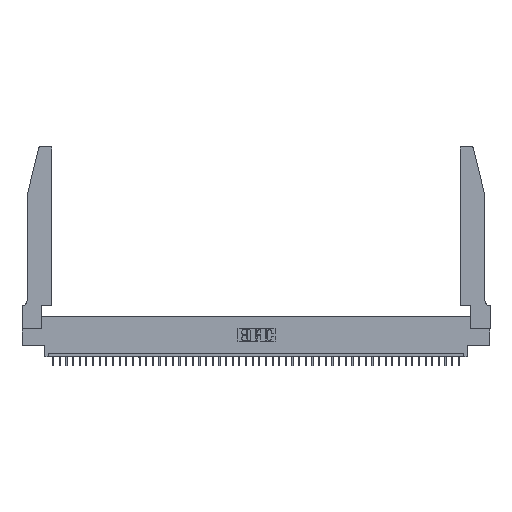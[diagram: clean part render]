
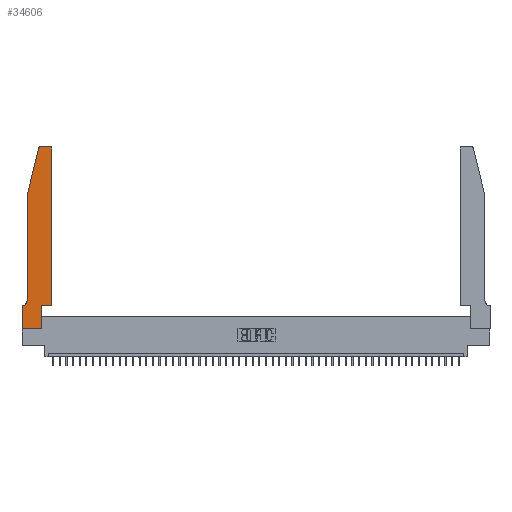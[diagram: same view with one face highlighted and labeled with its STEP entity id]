
A CAD part, top view. The second image highlights one B-rep face of the part: STEP entity #34606.
In plain terms, the highlighted planar face has unit normal (0, 0, 1).
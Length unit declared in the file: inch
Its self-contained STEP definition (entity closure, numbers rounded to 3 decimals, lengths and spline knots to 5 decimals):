
#27 = LINE ( 'NONE', #37163, #32215 ) ;
#949 = EDGE_CURVE ( 'NONE', #12019, #35945, #25805, .T. ) ;
#1623 = CARTESIAN_POINT ( 'NONE',  ( 0., 0., 0.37 ) ) ;
#2057 = EDGE_CURVE ( 'NONE', #35945, #33795, #44319, .T. ) ;
#2395 = CARTESIAN_POINT ( 'NONE',  ( 0.0055, 0.42, 0.37 ) ) ;
#2477 = CARTESIAN_POINT ( 'NONE',  ( 0., 0., 0.37 ) ) ;
#3123 = DIRECTION ( 'NONE',  ( 0., 0., -1. ) ) ;
#3147 = VERTEX_POINT ( 'NONE', #5386 ) ;
#3168 = EDGE_CURVE ( 'NONE', #45977, #38940, #31889, .T. ) ;
#3375 = VECTOR ( 'NONE', #35908, 39.37008 ) ;
#3614 = CARTESIAN_POINT ( 'NONE',  ( 0.25487, 2.72718, 0.37 ) ) ;
#4338 = VERTEX_POINT ( 'NONE', #19245 ) ;
#5386 = CARTESIAN_POINT ( 'NONE',  ( 0.2865, 0., 0.37 ) ) ;
#5485 = ORIENTED_EDGE ( 'NONE', *, *, #949, .T. ) ;
#5562 = DIRECTION ( 'NONE',  ( 0., 1., 0. ) ) ;
#5566 = AXIS2_PLACEMENT_3D ( 'NONE', #2395, #3123, #21718 ) ;
#6478 = DIRECTION ( 'NONE',  ( 0., -1., 0. ) ) ;
#6971 = LINE ( 'NONE', #25288, #21733 ) ;
#7958 = CARTESIAN_POINT ( 'NONE',  ( 0.0755, 0.35, 0.37 ) ) ;
#8302 = ORIENTED_EDGE ( 'NONE', *, *, #30953, .T. ) ;
#8475 = VECTOR ( 'NONE', #5562, 39.37008 ) ;
#9102 = ORIENTED_EDGE ( 'NONE', *, *, #42609, .T. ) ;
#9975 = FACE_OUTER_BOUND ( 'NONE', #25365, .T. ) ;
#11468 = VERTEX_POINT ( 'NONE', #31606 ) ;
#12019 = VERTEX_POINT ( 'NONE', #45371 ) ;
#12192 = DIRECTION ( 'NONE',  ( -1., 0., 0. ) ) ;
#12514 = CARTESIAN_POINT ( 'NONE',  ( 0., 0.35, 0.37 ) ) ;
#12577 = ORIENTED_EDGE ( 'NONE', *, *, #33414, .T. ) ;
#13039 = EDGE_CURVE ( 'NONE', #3147, #12019, #20422, .T. ) ;
#13443 = VECTOR ( 'NONE', #12192, 39.37008 ) ;
#14098 = DIRECTION ( 'NONE',  ( -1., 0., 0. ) ) ;
#14889 = VERTEX_POINT ( 'NONE', #1623 ) ;
#15368 = EDGE_CURVE ( 'NONE', #11468, #46173, #41874, .T. ) ;
#16467 = CARTESIAN_POINT ( 'NONE',  ( 0.2865, 0.35, 0.37 ) ) ;
#16618 = VERTEX_POINT ( 'NONE', #30522 ) ;
#16933 = DIRECTION ( 'NONE',  ( 0., 1., 0. ) ) ;
#17133 = AXIS2_PLACEMENT_3D ( 'NONE', #39086, #43073, #20307 ) ;
#17667 = EDGE_CURVE ( 'NONE', #16618, #11468, #26088, .T. ) ;
#17673 = ORIENTED_EDGE ( 'NONE', *, *, #17667, .T. ) ;
#18269 = ORIENTED_EDGE ( 'NONE', *, *, #13039, .T. ) ;
#19245 = CARTESIAN_POINT ( 'NONE',  ( 0.284, 2.75, 0.37 ) ) ;
#19582 = CARTESIAN_POINT ( 'NONE',  ( 0.4505, 0.35, 0.37 ) ) ;
#20307 = DIRECTION ( 'NONE',  ( 1., 0., 0. ) ) ;
#20358 = VECTOR ( 'NONE', #32283, 39.37008 ) ;
#20413 = CARTESIAN_POINT ( 'NONE',  ( 0.4205, 2.72, 0.37 ) ) ;
#20422 = LINE ( 'NONE', #16467, #8475 ) ;
#21428 = VECTOR ( 'NONE', #16933, 39.37008 ) ;
#21633 = CARTESIAN_POINT ( 'NONE',  ( 0.4505, 0.35, 0.37 ) ) ;
#21718 = DIRECTION ( 'NONE',  ( -1., 0., 0. ) ) ;
#21733 = VECTOR ( 'NONE', #6478, 39.37008 ) ;
#21983 = CARTESIAN_POINT ( 'NONE',  ( 0.4205, 2.75, 0.37 ) ) ;
#23377 = ORIENTED_EDGE ( 'NONE', *, *, #3168, .T. ) ;
#24182 = VERTEX_POINT ( 'NONE', #21983 ) ;
#25288 = CARTESIAN_POINT ( 'NONE',  ( 0.0755, 2., 0.37 ) ) ;
#25365 = EDGE_LOOP ( 'NONE', ( #9102, #8302, #23377, #39680, #17673, #28642, #37213, #12577, #18269, #5485, #45964, #38663 ) ) ;
#25805 = LINE ( 'NONE', #21633, #20358 ) ;
#25905 = CARTESIAN_POINT ( 'NONE',  ( 0.4505, 2.72, 0.37 ) ) ;
#26081 = AXIS2_PLACEMENT_3D ( 'NONE', #20413, #27859, #43182 ) ;
#26088 = CIRCLE ( 'NONE', #5566, 0.07 ) ;
#27859 = DIRECTION ( 'NONE',  ( 0., 0., 1. ) ) ;
#28500 = LINE ( 'NONE', #2477, #3375 ) ;
#28642 = ORIENTED_EDGE ( 'NONE', *, *, #15368, .T. ) ;
#30522 = CARTESIAN_POINT ( 'NONE',  ( 0.0755, 0.42, 0.37 ) ) ;
#30773 = VECTOR ( 'NONE', #14098, 39.37008 ) ;
#30953 = EDGE_CURVE ( 'NONE', #4338, #45977, #38408, .T. ) ;
#31606 = CARTESIAN_POINT ( 'NONE',  ( 0.0055, 0.35, 0.37 ) ) ;
#31876 = EDGE_CURVE ( 'NONE', #46173, #14889, #27, .T. ) ;
#31889 = LINE ( 'NONE', #42284, #40995 ) ;
#32215 = VECTOR ( 'NONE', #44355, 39.37008 ) ;
#32283 = DIRECTION ( 'NONE',  ( 1., 0., 0. ) ) ;
#32893 = CARTESIAN_POINT ( 'NONE',  ( 0.2605, 2.75, 0.37 ) ) ;
#33414 = EDGE_CURVE ( 'NONE', #14889, #3147, #28500, .T. ) ;
#33795 = VERTEX_POINT ( 'NONE', #25905 ) ;
#34606 = ADVANCED_FACE ( 'NONE', ( #9975 ), #44114, .T. ) ;
#35763 = EDGE_CURVE ( 'NONE', #38940, #16618, #6971, .T. ) ;
#35908 = DIRECTION ( 'NONE',  ( 1., 0., 0. ) ) ;
#35945 = VERTEX_POINT ( 'NONE', #19582 ) ;
#37163 = CARTESIAN_POINT ( 'NONE',  ( 0., 0., 0.37 ) ) ;
#37213 = ORIENTED_EDGE ( 'NONE', *, *, #31876, .T. ) ;
#37334 = LINE ( 'NONE', #32893, #30773 ) ;
#38408 = CIRCLE ( 'NONE', #17133, 0.03 ) ;
#38663 = ORIENTED_EDGE ( 'NONE', *, *, #43813, .T. ) ;
#38940 = VERTEX_POINT ( 'NONE', #46701 ) ;
#39086 = CARTESIAN_POINT ( 'NONE',  ( 0.284, 2.72, 0.37 ) ) ;
#39680 = ORIENTED_EDGE ( 'NONE', *, *, #35763, .T. ) ;
#39838 = AXIS2_PLACEMENT_3D ( 'NONE', #44608, #40395, #47856 ) ;
#40395 = DIRECTION ( 'NONE',  ( 0., 0., 1. ) ) ;
#40995 = VECTOR ( 'NONE', #46998, 39.37008 ) ;
#41092 = CIRCLE ( 'NONE', #26081, 0.03 ) ;
#41874 = LINE ( 'NONE', #7958, #13443 ) ;
#42284 = CARTESIAN_POINT ( 'NONE',  ( 0.0755, 2., 0.37 ) ) ;
#42609 = EDGE_CURVE ( 'NONE', #24182, #4338, #37334, .T. ) ;
#43073 = DIRECTION ( 'NONE',  ( 0., 0., 1. ) ) ;
#43182 = DIRECTION ( 'NONE',  ( 1., 0., 0. ) ) ;
#43813 = EDGE_CURVE ( 'NONE', #33795, #24182, #41092, .T. ) ;
#44114 = PLANE ( 'NONE',  #39838 ) ;
#44319 = LINE ( 'NONE', #48050, #21428 ) ;
#44355 = DIRECTION ( 'NONE',  ( 0., -1., 0. ) ) ;
#44608 = CARTESIAN_POINT ( 'NONE',  ( 0., 0.35, 0.37 ) ) ;
#45371 = CARTESIAN_POINT ( 'NONE',  ( 0.2865, 0.35, 0.37 ) ) ;
#45964 = ORIENTED_EDGE ( 'NONE', *, *, #2057, .T. ) ;
#45977 = VERTEX_POINT ( 'NONE', #3614 ) ;
#46173 = VERTEX_POINT ( 'NONE', #12514 ) ;
#46701 = CARTESIAN_POINT ( 'NONE',  ( 0.0755, 2., 0.37 ) ) ;
#46998 = DIRECTION ( 'NONE',  ( -0.239, -0.971, 0. ) ) ;
#47856 = DIRECTION ( 'NONE',  ( 1., 0., 0. ) ) ;
#48050 = CARTESIAN_POINT ( 'NONE',  ( 0.4505, 0.35, 0.37 ) ) ;
